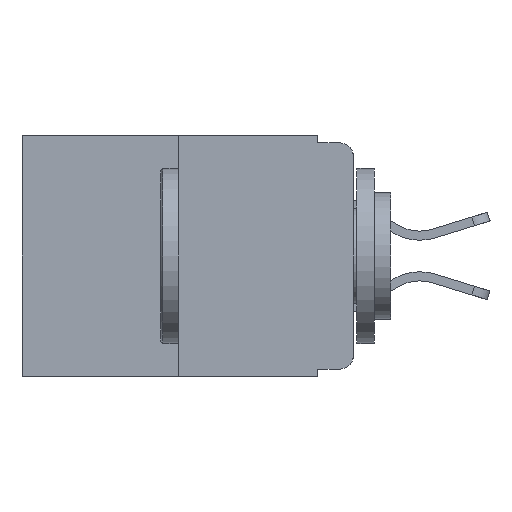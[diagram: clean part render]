
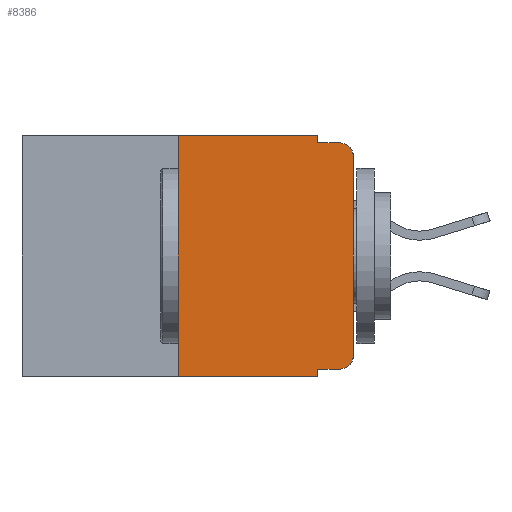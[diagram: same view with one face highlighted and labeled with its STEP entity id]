
A CAD part, left-side view. The second image highlights one B-rep face of the part: STEP entity #8386.
In plain terms, the highlighted planar face has unit normal (-1, 0, 0).
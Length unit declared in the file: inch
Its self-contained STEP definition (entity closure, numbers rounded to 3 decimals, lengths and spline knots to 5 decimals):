
#51 = DIRECTION ( 'NONE',  ( 0., -1., 0. ) ) ;
#160 = VERTEX_POINT ( 'NONE', #181 ) ;
#171 = ORIENTED_EDGE ( 'NONE', *, *, #8788, .T. ) ;
#181 = CARTESIAN_POINT ( 'NONE',  ( 0., 0., -0.03 ) ) ;
#204 = CARTESIAN_POINT ( 'NONE',  ( 0., 0.25, 0. ) ) ;
#387 = DIRECTION ( 'NONE',  ( -1., 0., 0. ) ) ;
#418 = CARTESIAN_POINT ( 'NONE',  ( 0., 0.051, -0.343 ) ) ;
#580 = DIRECTION ( 'NONE',  ( 0., 0., -1. ) ) ;
#588 = VERTEX_POINT ( 'NONE', #7911 ) ;
#603 = VERTEX_POINT ( 'NONE', #5504 ) ;
#767 = DIRECTION ( 'NONE',  ( 0., 0., -1. ) ) ;
#795 = AXIS2_PLACEMENT_3D ( 'NONE', #8913, #7112, #1366 ) ;
#830 = CARTESIAN_POINT ( 'NONE',  ( 0., 0.25, -0.343 ) ) ;
#867 = VERTEX_POINT ( 'NONE', #418 ) ;
#1038 = LINE ( 'NONE', #7701, #6161 ) ;
#1366 = DIRECTION ( 'NONE',  ( 0., 0., -1. ) ) ;
#1593 = DIRECTION ( 'NONE',  ( -1., 0., 0. ) ) ;
#1865 = ORIENTED_EDGE ( 'NONE', *, *, #10414, .F. ) ;
#1988 = AXIS2_PLACEMENT_3D ( 'NONE', #7329, #1593, #8237 ) ;
#2085 = DIRECTION ( 'NONE',  ( 0., 0., 1. ) ) ;
#2284 = DIRECTION ( 'NONE',  ( 0., 0., 1. ) ) ;
#2364 = AXIS2_PLACEMENT_3D ( 'NONE', #6190, #387, #7137 ) ;
#2447 = VECTOR ( 'NONE', #51, 39.37008 ) ;
#2928 = ORIENTED_EDGE ( 'NONE', *, *, #11287, .F. ) ;
#3016 = FACE_OUTER_BOUND ( 'NONE', #9622, .T. ) ;
#3275 = PLANE ( 'NONE',  #795 ) ;
#3277 = LINE ( 'NONE', #204, #7721 ) ;
#3344 = EDGE_CURVE ( 'NONE', #8154, #10213, #3277, .T. ) ;
#3439 = VERTEX_POINT ( 'NONE', #7100 ) ;
#3524 = CARTESIAN_POINT ( 'NONE',  ( 0., 0.473, -0.343 ) ) ;
#3666 = ORIENTED_EDGE ( 'NONE', *, *, #9465, .T. ) ;
#3708 = VECTOR ( 'NONE', #2085, 39.37008 ) ;
#3850 = VERTEX_POINT ( 'NONE', #10825 ) ;
#3969 = ORIENTED_EDGE ( 'NONE', *, *, #5111, .T. ) ;
#4440 = CIRCLE ( 'NONE', #2364, 0.02 ) ;
#4442 = LINE ( 'NONE', #11891, #9117 ) ;
#4872 = DIRECTION ( 'NONE',  ( 0., -1., 0. ) ) ;
#4893 = CARTESIAN_POINT ( 'NONE',  ( 0., 0.051, -0.01 ) ) ;
#4999 = VERTEX_POINT ( 'NONE', #10515 ) ;
#5017 = CARTESIAN_POINT ( 'NONE',  ( 0., 0., 0. ) ) ;
#5111 = EDGE_CURVE ( 'NONE', #160, #4999, #4440, .T. ) ;
#5206 = CARTESIAN_POINT ( 'NONE',  ( 0., 0.25, 0. ) ) ;
#5317 = LINE ( 'NONE', #4893, #2447 ) ;
#5504 = CARTESIAN_POINT ( 'NONE',  ( 0., 0.051, -0.01 ) ) ;
#5517 = EDGE_CURVE ( 'NONE', #603, #4999, #5317, .T. ) ;
#6161 = VECTOR ( 'NONE', #4872, 39.37008 ) ;
#6190 = CARTESIAN_POINT ( 'NONE',  ( 0., 0.02, -0.03 ) ) ;
#6622 = CARTESIAN_POINT ( 'NONE',  ( 0., 0.473, 0. ) ) ;
#6639 = LINE ( 'NONE', #3524, #11667 ) ;
#6688 = ORIENTED_EDGE ( 'NONE', *, *, #8033, .T. ) ;
#6727 = CARTESIAN_POINT ( 'NONE',  ( 0., 0.051, 0. ) ) ;
#7100 = CARTESIAN_POINT ( 'NONE',  ( 0., 0.051, -0.333 ) ) ;
#7112 = DIRECTION ( 'NONE',  ( 1., 0., 0. ) ) ;
#7137 = DIRECTION ( 'NONE',  ( 0., 0., -1. ) ) ;
#7176 = EDGE_CURVE ( 'NONE', #588, #3850, #11265, .T. ) ;
#7329 = CARTESIAN_POINT ( 'NONE',  ( 0., 0.02, -0.313 ) ) ;
#7426 = VERTEX_POINT ( 'NONE', #6727 ) ;
#7701 = CARTESIAN_POINT ( 'NONE',  ( 0., 0.051, -0.333 ) ) ;
#7721 = VECTOR ( 'NONE', #2284, 39.37008 ) ;
#7807 = ORIENTED_EDGE ( 'NONE', *, *, #7176, .T. ) ;
#7911 = CARTESIAN_POINT ( 'NONE',  ( 0., 0.02, -0.333 ) ) ;
#8033 = EDGE_CURVE ( 'NONE', #8154, #867, #6639, .T. ) ;
#8154 = VERTEX_POINT ( 'NONE', #830 ) ;
#8237 = DIRECTION ( 'NONE',  ( 0., 0., -1. ) ) ;
#8243 = ORIENTED_EDGE ( 'NONE', *, *, #3344, .F. ) ;
#8386 = ADVANCED_FACE ( 'NONE', ( #3016 ), #3275, .F. ) ;
#8430 = LINE ( 'NONE', #5017, #3708 ) ;
#8788 = EDGE_CURVE ( 'NONE', #3439, #588, #1038, .T. ) ;
#8913 = CARTESIAN_POINT ( 'NONE',  ( 0., 0.473, 0. ) ) ;
#8968 = LINE ( 'NONE', #6622, #11573 ) ;
#9117 = VECTOR ( 'NONE', #767, 39.37008 ) ;
#9252 = VECTOR ( 'NONE', #580, 39.37008 ) ;
#9465 = EDGE_CURVE ( 'NONE', #3850, #160, #8430, .T. ) ;
#9622 = EDGE_LOOP ( 'NONE', ( #3666, #3969, #11844, #9791, #2928, #8243, #6688, #1865, #171, #7807 ) ) ;
#9791 = ORIENTED_EDGE ( 'NONE', *, *, #10630, .F. ) ;
#10038 = DIRECTION ( 'NONE',  ( 0., -1., 0. ) ) ;
#10211 = DIRECTION ( 'NONE',  ( 0., -1., 0. ) ) ;
#10213 = VERTEX_POINT ( 'NONE', #5206 ) ;
#10414 = EDGE_CURVE ( 'NONE', #3439, #867, #4442, .T. ) ;
#10515 = CARTESIAN_POINT ( 'NONE',  ( 0., 0.02, -0.01 ) ) ;
#10630 = EDGE_CURVE ( 'NONE', #7426, #603, #11571, .T. ) ;
#10825 = CARTESIAN_POINT ( 'NONE',  ( 0., 0., -0.313 ) ) ;
#10861 = CARTESIAN_POINT ( 'NONE',  ( 0., 0.051, 0. ) ) ;
#11265 = CIRCLE ( 'NONE', #1988, 0.02 ) ;
#11287 = EDGE_CURVE ( 'NONE', #10213, #7426, #8968, .T. ) ;
#11571 = LINE ( 'NONE', #10861, #9252 ) ;
#11573 = VECTOR ( 'NONE', #10211, 39.37008 ) ;
#11667 = VECTOR ( 'NONE', #10038, 39.37008 ) ;
#11844 = ORIENTED_EDGE ( 'NONE', *, *, #5517, .F. ) ;
#11891 = CARTESIAN_POINT ( 'NONE',  ( 0., 0.051, 0. ) ) ;
